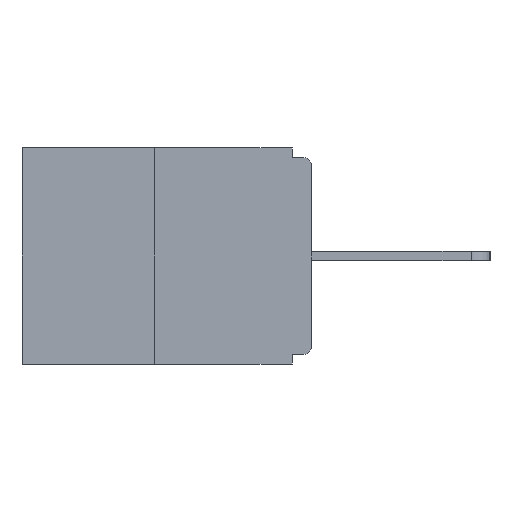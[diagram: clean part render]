
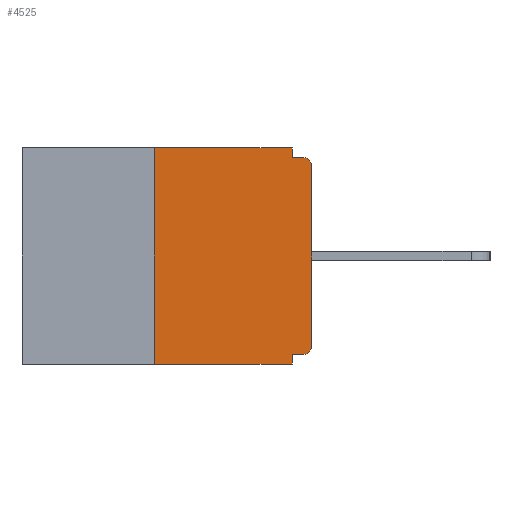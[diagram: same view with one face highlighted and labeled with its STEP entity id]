
A CAD part, left-side view. The second image highlights one B-rep face of the part: STEP entity #4525.
In plain terms, the highlighted planar face has unit normal (-1, 0, 0).
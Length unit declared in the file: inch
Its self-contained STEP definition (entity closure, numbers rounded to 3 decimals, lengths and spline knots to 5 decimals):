
#298 = CARTESIAN_POINT ( 'NONE',  ( 0., 0.031, -0.015 ) ) ;
#701 = DIRECTION ( 'NONE',  ( 0., 0., -1. ) ) ;
#2664 = CARTESIAN_POINT ( 'NONE',  ( 0., 0.015, -0.015 ) ) ;
#2736 = ORIENTED_EDGE ( 'NONE', *, *, #23784, .F. ) ;
#2839 = DIRECTION ( 'NONE',  ( 0., 1., 0. ) ) ;
#3126 = CARTESIAN_POINT ( 'NONE',  ( 0., 0.46, -0.343 ) ) ;
#3641 = VERTEX_POINT ( 'NONE', #11613 ) ;
#3755 = CARTESIAN_POINT ( 'NONE',  ( 0., 0., -0.03 ) ) ;
#4232 = CARTESIAN_POINT ( 'NONE',  ( 0., 0., -0.313 ) ) ;
#4360 = AXIS2_PLACEMENT_3D ( 'NONE', #13755, #4560, #701 ) ;
#4525 = ADVANCED_FACE ( 'NONE', ( #4911 ), #14854, .F. ) ;
#4560 = DIRECTION ( 'NONE',  ( -1., 0., 0. ) ) ;
#4704 = VECTOR ( 'NONE', #13064, 39.37008 ) ;
#4818 = VERTEX_POINT ( 'NONE', #6906 ) ;
#4826 = LINE ( 'NONE', #23997, #24600 ) ;
#4911 = FACE_OUTER_BOUND ( 'NONE', #13208, .T. ) ;
#5001 = AXIS2_PLACEMENT_3D ( 'NONE', #24010, #11877, #26044 ) ;
#5062 = ORIENTED_EDGE ( 'NONE', *, *, #10202, .F. ) ;
#5177 = EDGE_CURVE ( 'NONE', #15810, #17183, #14786, .T. ) ;
#5195 = DIRECTION ( 'NONE',  ( 0., -1., 0. ) ) ;
#5257 = CARTESIAN_POINT ( 'NONE',  ( 0., 0., 0. ) ) ;
#5424 = EDGE_CURVE ( 'NONE', #18272, #7385, #19798, .T. ) ;
#6326 = ORIENTED_EDGE ( 'NONE', *, *, #13277, .F. ) ;
#6662 = ORIENTED_EDGE ( 'NONE', *, *, #14942, .T. ) ;
#6906 = CARTESIAN_POINT ( 'NONE',  ( 0., 0.031, 0. ) ) ;
#7385 = VERTEX_POINT ( 'NONE', #4232 ) ;
#7593 = ORIENTED_EDGE ( 'NONE', *, *, #15918, .F. ) ;
#8542 = ORIENTED_EDGE ( 'NONE', *, *, #14204, .T. ) ;
#8652 = AXIS2_PLACEMENT_3D ( 'NONE', #15538, #15386, #17367 ) ;
#8704 = CARTESIAN_POINT ( 'NONE',  ( 0., 0.031, -0.328 ) ) ;
#9393 = VECTOR ( 'NONE', #10099, 39.37008 ) ;
#10099 = DIRECTION ( 'NONE',  ( 0., -1., 0. ) ) ;
#10202 = EDGE_CURVE ( 'NONE', #4818, #15810, #4826, .T. ) ;
#10322 = LINE ( 'NONE', #3126, #20384 ) ;
#10476 = EDGE_CURVE ( 'NONE', #23303, #21137, #23609, .T. ) ;
#11065 = CARTESIAN_POINT ( 'NONE',  ( 0., 0.031, -0.343 ) ) ;
#11613 = CARTESIAN_POINT ( 'NONE',  ( 0., 0.031, -0.343 ) ) ;
#11877 = DIRECTION ( 'NONE',  ( -1., 0., 0. ) ) ;
#11921 = VECTOR ( 'NONE', #14146, 39.37008 ) ;
#12515 = DIRECTION ( 'NONE',  ( 0., 0., 1. ) ) ;
#12687 = CARTESIAN_POINT ( 'NONE',  ( 0., 0.25, 0. ) ) ;
#12695 = ORIENTED_EDGE ( 'NONE', *, *, #10476, .F. ) ;
#12870 = VECTOR ( 'NONE', #2839, 39.37008 ) ;
#13064 = DIRECTION ( 'NONE',  ( 0., 0., -1. ) ) ;
#13208 = EDGE_LOOP ( 'NONE', ( #2736, #12695, #8542, #7593, #6326, #14954, #6662, #24824, #20633, #5062 ) ) ;
#13277 = EDGE_CURVE ( 'NONE', #18272, #14046, #13517, .T. ) ;
#13517 = LINE ( 'NONE', #15098, #12870 ) ;
#13755 = CARTESIAN_POINT ( 'NONE',  ( 0., 0.015, -0.313 ) ) ;
#14046 = VERTEX_POINT ( 'NONE', #8704 ) ;
#14062 = LINE ( 'NONE', #5257, #24860 ) ;
#14146 = DIRECTION ( 'NONE',  ( 0., -1., 0. ) ) ;
#14204 = EDGE_CURVE ( 'NONE', #23303, #3641, #10322, .T. ) ;
#14786 = LINE ( 'NONE', #25240, #9393 ) ;
#14854 = PLANE ( 'NONE',  #8652 ) ;
#14942 = EDGE_CURVE ( 'NONE', #7385, #23757, #14062, .T. ) ;
#14954 = ORIENTED_EDGE ( 'NONE', *, *, #5424, .T. ) ;
#15098 = CARTESIAN_POINT ( 'NONE',  ( 0., 0., -0.328 ) ) ;
#15386 = DIRECTION ( 'NONE',  ( 1., 0., 0. ) ) ;
#15538 = CARTESIAN_POINT ( 'NONE',  ( 0., 0.46, 0. ) ) ;
#15784 = CIRCLE ( 'NONE', #5001, 0.015 ) ;
#15810 = VERTEX_POINT ( 'NONE', #298 ) ;
#15918 = EDGE_CURVE ( 'NONE', #14046, #3641, #20929, .T. ) ;
#16962 = CARTESIAN_POINT ( 'NONE',  ( 0., 0.25, 0. ) ) ;
#17183 = VERTEX_POINT ( 'NONE', #2664 ) ;
#17272 = LINE ( 'NONE', #22171, #11921 ) ;
#17367 = DIRECTION ( 'NONE',  ( 0., 0., -1. ) ) ;
#17450 = DIRECTION ( 'NONE',  ( 0., 0., 1. ) ) ;
#18155 = VECTOR ( 'NONE', #12515, 39.37008 ) ;
#18272 = VERTEX_POINT ( 'NONE', #21040 ) ;
#18543 = EDGE_CURVE ( 'NONE', #23757, #17183, #15784, .T. ) ;
#19798 = CIRCLE ( 'NONE', #4360, 0.015 ) ;
#20384 = VECTOR ( 'NONE', #5195, 39.37008 ) ;
#20503 = CARTESIAN_POINT ( 'NONE',  ( 0., 0.25, -0.343 ) ) ;
#20633 = ORIENTED_EDGE ( 'NONE', *, *, #5177, .F. ) ;
#20929 = LINE ( 'NONE', #11065, #4704 ) ;
#21040 = CARTESIAN_POINT ( 'NONE',  ( 0., 0.015, -0.328 ) ) ;
#21137 = VERTEX_POINT ( 'NONE', #16962 ) ;
#22171 = CARTESIAN_POINT ( 'NONE',  ( 0., 0.46, 0. ) ) ;
#23303 = VERTEX_POINT ( 'NONE', #20503 ) ;
#23609 = LINE ( 'NONE', #12687, #18155 ) ;
#23636 = DIRECTION ( 'NONE',  ( 0., 0., -1. ) ) ;
#23757 = VERTEX_POINT ( 'NONE', #3755 ) ;
#23784 = EDGE_CURVE ( 'NONE', #21137, #4818, #17272, .T. ) ;
#23997 = CARTESIAN_POINT ( 'NONE',  ( 0., 0.031, 0. ) ) ;
#24010 = CARTESIAN_POINT ( 'NONE',  ( 0., 0.015, -0.03 ) ) ;
#24600 = VECTOR ( 'NONE', #23636, 39.37008 ) ;
#24824 = ORIENTED_EDGE ( 'NONE', *, *, #18543, .T. ) ;
#24860 = VECTOR ( 'NONE', #17450, 39.37008 ) ;
#25240 = CARTESIAN_POINT ( 'NONE',  ( 0., 0., -0.015 ) ) ;
#26044 = DIRECTION ( 'NONE',  ( 0., 0., -1. ) ) ;
